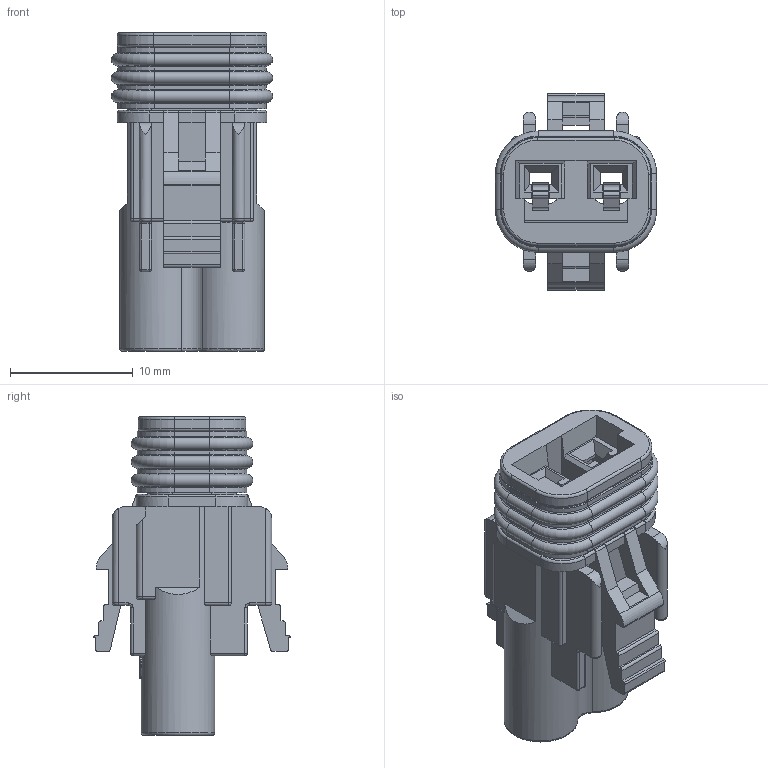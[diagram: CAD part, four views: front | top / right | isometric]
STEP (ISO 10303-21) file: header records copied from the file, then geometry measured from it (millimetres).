
FILE_DESCRIPTION (( 'STEP AP214' ), '1' );
FILE_NAME ('572-002-000-400.STEP', '2020-07-30T18:28:14', ( '' ), ( '' ), 'SwSTEP 2.0', 'SolidWorks 2020', '' );
FILE_SCHEMA (( 'AUTOMOTIVE_DESIGN' ));
Length unit declared in the file: millimetre
Products named in the file (3): 572-002-000-FEMALE-HOUSING_BLUE; 572-002-000-400; 570-002-000-HOUSING-SEAL
Assembly tree (2 placements, depth 2):
  572-002-000-400
    572-002-000-FEMALE-HOUSING_BLUE
    570-002-000-HOUSING-SEAL
Bounding box: 13.15 x 16 x 26 mm (x, y, z)
Volume: 1445.7 mm3; surface area: 3154.6 mm2
Topology: 2 solids, 4 shells, 692 faces, 1733 edges, 1040 vertices
Faces by surface type: plane 307, cylinder 247, torus 114, sphere 10, bspline 8, cone 6
Entity records: 20804 total; most frequent: CARTESIAN_POINT 4090, DIRECTION 3597, ORIENTED_EDGE 3446, EDGE_CURVE 1723, AXIS2_PLACEMENT_3D 1298, VERTEX_POINT 1040, VECTOR 1001, LINE 1001
